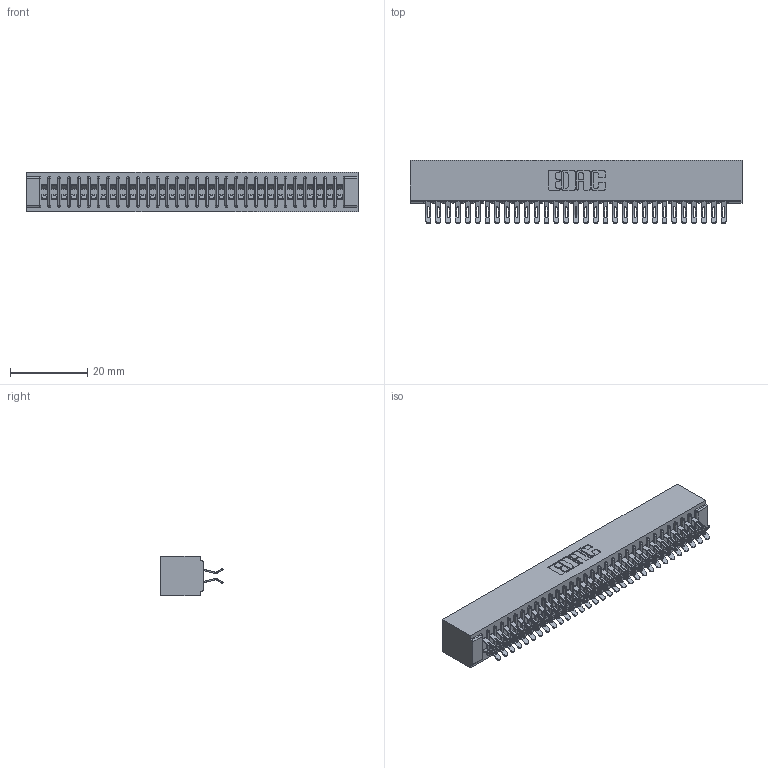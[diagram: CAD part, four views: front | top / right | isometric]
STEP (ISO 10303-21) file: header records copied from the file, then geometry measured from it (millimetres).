
FILE_DESCRIPTION (( 'STEP AP203' ), '1' );
FILE_NAME ('341-062-555-201.STEP', '2018-08-07T17:57:41', ( '' ), ( '' ), 'SwSTEP 2.0', 'SolidWorks 2016', '' );
FILE_SCHEMA (( 'CONFIG_CONTROL_DESIGN' ));
Length unit declared in the file: inch
Products named in the file (3): 341-292-001_341-292-155; 341-062-555-201; 341 Part_No Mounting Lugs
Assembly tree (63 placements, depth 2):
  341-062-555-201
    341 Part_No Mounting Lugs
    341-292-001_341-292-155  x62
Bounding box: 85.72 x 16.31 x 10.16 mm (x, y, z)
Volume: 6635.3 mm3; surface area: 12599.5 mm2
Topology: 63 solids, 63 shells, 4944 faces, 14769 edges, 9614 vertices
Faces by surface type: plane 2668, cylinder 2152, sphere 64, torus 60
Entity records: 39174 total; most frequent: CARTESIAN_POINT 6527, ORIENTED_EDGE 6474, DIRECTION 6331, EDGE_CURVE 3237, LINE 2591, VECTOR 2591, VERTEX_POINT 2050, AXIS2_PLACEMENT_3D 1870
